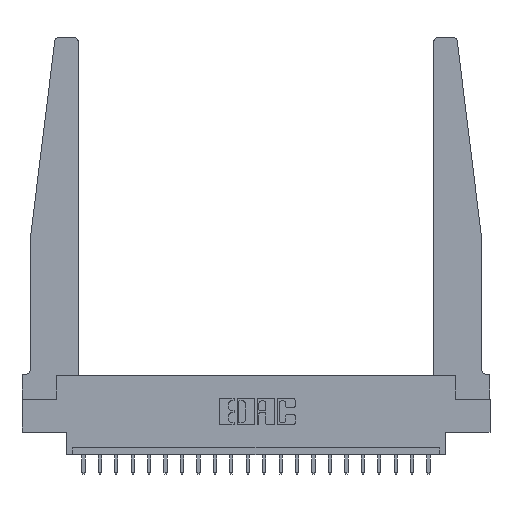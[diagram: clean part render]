
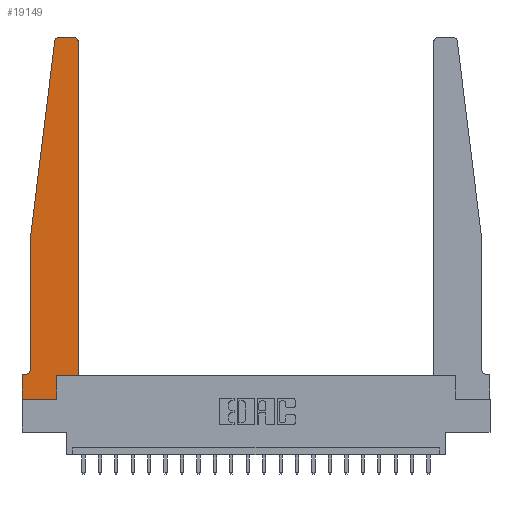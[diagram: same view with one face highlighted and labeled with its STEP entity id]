
A CAD part, top view. The second image highlights one B-rep face of the part: STEP entity #19149.
In plain terms, the highlighted planar face has unit normal (0, 0, 1).
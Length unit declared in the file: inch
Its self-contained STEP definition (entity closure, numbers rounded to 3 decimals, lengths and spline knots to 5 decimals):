
#135 = DIRECTION ( 'NONE',  ( 0., -1., 0. ) ) ;
#217 = ORIENTED_EDGE ( 'NONE', *, *, #11594, .T. ) ;
#1072 = EDGE_CURVE ( 'NONE', #12486, #4913, #5628, .T. ) ;
#1223 = ORIENTED_EDGE ( 'NONE', *, *, #2847, .T. ) ;
#1308 = CARTESIAN_POINT ( 'NONE',  ( 0.065, 0.2375, 0.37 ) ) ;
#1382 = LINE ( 'NONE', #15746, #2912 ) ;
#1485 = LINE ( 'NONE', #18086, #12271 ) ;
#2259 = EDGE_CURVE ( 'NONE', #8871, #21013, #1382, .T. ) ;
#2644 = VECTOR ( 'NONE', #6236, 39.37008 ) ;
#2665 = DIRECTION ( 'NONE',  ( 1., 0., 0. ) ) ;
#2669 = AXIS2_PLACEMENT_3D ( 'NONE', #3501, #15025, #10392 ) ;
#2847 = EDGE_CURVE ( 'NONE', #19261, #7561, #9054, .T. ) ;
#2912 = VECTOR ( 'NONE', #2665, 39.37008 ) ;
#3026 = EDGE_CURVE ( 'NONE', #7064, #3245, #9560, .T. ) ;
#3198 = CARTESIAN_POINT ( 'NONE',  ( 0.24675, 2.72367, 0.37 ) ) ;
#3245 = VERTEX_POINT ( 'NONE', #12214 ) ;
#3501 = CARTESIAN_POINT ( 'NONE',  ( 0.27653, 2.72, 0.37 ) ) ;
#4122 = LINE ( 'NONE', #7102, #8521 ) ;
#4364 = CARTESIAN_POINT ( 'NONE',  ( 0.425, 0.18, 0.37 ) ) ;
#4913 = VERTEX_POINT ( 'NONE', #14708 ) ;
#4915 = DIRECTION ( 'NONE',  ( 0., 0., -1. ) ) ;
#5219 = VERTEX_POINT ( 'NONE', #1308 ) ;
#5628 = LINE ( 'NONE', #20879, #20015 ) ;
#6236 = DIRECTION ( 'NONE',  ( 0., 1., 0. ) ) ;
#6608 = ORIENTED_EDGE ( 'NONE', *, *, #3026, .T. ) ;
#6742 = VECTOR ( 'NONE', #10210, 39.37008 ) ;
#6780 = ORIENTED_EDGE ( 'NONE', *, *, #20189, .T. ) ;
#7064 = VERTEX_POINT ( 'NONE', #3198 ) ;
#7102 = CARTESIAN_POINT ( 'NONE',  ( 0.065, 0.1875, 0.37 ) ) ;
#7144 = CARTESIAN_POINT ( 'NONE',  ( 0.425, 2.72, 0.37 ) ) ;
#7561 = VERTEX_POINT ( 'NONE', #20354 ) ;
#7652 = AXIS2_PLACEMENT_3D ( 'NONE', #14944, #11696, #16441 ) ;
#7834 = ORIENTED_EDGE ( 'NONE', *, *, #17759, .T. ) ;
#8238 = DIRECTION ( 'NONE',  ( 1., 0., 0. ) ) ;
#8492 = CARTESIAN_POINT ( 'NONE',  ( 0.015, 0.1875, 0.37 ) ) ;
#8521 = VECTOR ( 'NONE', #11945, 39.37008 ) ;
#8651 = EDGE_CURVE ( 'NONE', #21013, #19261, #9976, .T. ) ;
#8871 = VERTEX_POINT ( 'NONE', #14206 ) ;
#8902 = EDGE_CURVE ( 'NONE', #5219, #15879, #19164, .T. ) ;
#9054 = CIRCLE ( 'NONE', #15491, 0.03 ) ;
#9259 = DIRECTION ( 'NONE',  ( -1., 0., 0. ) ) ;
#9560 = LINE ( 'NONE', #20122, #6742 ) ;
#9637 = ORIENTED_EDGE ( 'NONE', *, *, #8902, .T. ) ;
#9726 = VECTOR ( 'NONE', #12309, 39.37008 ) ;
#9873 = DIRECTION ( 'NONE',  ( 0., 0., 1. ) ) ;
#9933 = DIRECTION ( 'NONE',  ( -1., 0., 0. ) ) ;
#9976 = LINE ( 'NONE', #10567, #9726 ) ;
#10210 = DIRECTION ( 'NONE',  ( -0.122, -0.992, 0. ) ) ;
#10392 = DIRECTION ( 'NONE',  ( 1., 0., 0. ) ) ;
#10567 = CARTESIAN_POINT ( 'NONE',  ( 0.425, 0.18, 0.37 ) ) ;
#11040 = LINE ( 'NONE', #17439, #18971 ) ;
#11268 = EDGE_CURVE ( 'NONE', #4913, #8871, #11399, .T. ) ;
#11399 = LINE ( 'NONE', #12800, #2644 ) ;
#11484 = PLANE ( 'NONE',  #7652 ) ;
#11594 = EDGE_CURVE ( 'NONE', #18854, #12486, #19063, .T. ) ;
#11696 = DIRECTION ( 'NONE',  ( 0., 0., 1. ) ) ;
#11792 = DIRECTION ( 'NONE',  ( 0., -1., 0. ) ) ;
#11945 = DIRECTION ( 'NONE',  ( -1., 0., 0. ) ) ;
#12076 = FACE_OUTER_BOUND ( 'NONE', #20095, .T. ) ;
#12214 = CARTESIAN_POINT ( 'NONE',  ( 0.065, 1.25, 0.37 ) ) ;
#12271 = VECTOR ( 'NONE', #11792, 39.37008 ) ;
#12309 = DIRECTION ( 'NONE',  ( 0., 1., 0. ) ) ;
#12486 = VERTEX_POINT ( 'NONE', #14514 ) ;
#12800 = CARTESIAN_POINT ( 'NONE',  ( 0.2605, 0.18, 0.37 ) ) ;
#13086 = VERTEX_POINT ( 'NONE', #14207 ) ;
#13185 = VECTOR ( 'NONE', #135, 39.37008 ) ;
#13651 = AXIS2_PLACEMENT_3D ( 'NONE', #15060, #4915, #9933 ) ;
#13880 = EDGE_CURVE ( 'NONE', #13086, #7064, #18957, .T. ) ;
#14080 = ORIENTED_EDGE ( 'NONE', *, *, #8651, .T. ) ;
#14206 = CARTESIAN_POINT ( 'NONE',  ( 0.2605, 0.18, 0.37 ) ) ;
#14207 = CARTESIAN_POINT ( 'NONE',  ( 0.27653, 2.75, 0.37 ) ) ;
#14514 = CARTESIAN_POINT ( 'NONE',  ( 0., 0., 0.37 ) ) ;
#14708 = CARTESIAN_POINT ( 'NONE',  ( 0.2605, 0., 0.37 ) ) ;
#14864 = ORIENTED_EDGE ( 'NONE', *, *, #1072, .T. ) ;
#14944 = CARTESIAN_POINT ( 'NONE',  ( 0., 0.1875, 0.37 ) ) ;
#15025 = DIRECTION ( 'NONE',  ( 0., 0., 1. ) ) ;
#15060 = CARTESIAN_POINT ( 'NONE',  ( 0.015, 0.2375, 0.37 ) ) ;
#15491 = AXIS2_PLACEMENT_3D ( 'NONE', #17991, #9873, #8238 ) ;
#15746 = CARTESIAN_POINT ( 'NONE',  ( 0.425, 0.18, 0.37 ) ) ;
#15879 = VERTEX_POINT ( 'NONE', #8492 ) ;
#16026 = ORIENTED_EDGE ( 'NONE', *, *, #18892, .T. ) ;
#16127 = DIRECTION ( 'NONE',  ( 1., 0., 0. ) ) ;
#16441 = DIRECTION ( 'NONE',  ( 1., 0., 0. ) ) ;
#16693 = CARTESIAN_POINT ( 'NONE',  ( 0., 0., 0.37 ) ) ;
#16878 = ORIENTED_EDGE ( 'NONE', *, *, #11268, .T. ) ;
#17439 = CARTESIAN_POINT ( 'NONE',  ( 0.25, 2.75, 0.37 ) ) ;
#17759 = EDGE_CURVE ( 'NONE', #15879, #18854, #4122, .T. ) ;
#17866 = ORIENTED_EDGE ( 'NONE', *, *, #13880, .T. ) ;
#17991 = CARTESIAN_POINT ( 'NONE',  ( 0.395, 2.72, 0.37 ) ) ;
#18086 = CARTESIAN_POINT ( 'NONE',  ( 0.065, 1.25, 0.37 ) ) ;
#18854 = VERTEX_POINT ( 'NONE', #19252 ) ;
#18892 = EDGE_CURVE ( 'NONE', #7561, #13086, #11040, .T. ) ;
#18957 = CIRCLE ( 'NONE', #2669, 0.03 ) ;
#18971 = VECTOR ( 'NONE', #9259, 39.37008 ) ;
#19063 = LINE ( 'NONE', #16693, #13185 ) ;
#19149 = ADVANCED_FACE ( 'NONE', ( #12076 ), #11484, .T. ) ;
#19164 = CIRCLE ( 'NONE', #13651, 0.05 ) ;
#19252 = CARTESIAN_POINT ( 'NONE',  ( 0., 0.1875, 0.37 ) ) ;
#19261 = VERTEX_POINT ( 'NONE', #7144 ) ;
#20015 = VECTOR ( 'NONE', #16127, 39.37008 ) ;
#20095 = EDGE_LOOP ( 'NONE', ( #16026, #17866, #6608, #6780, #9637, #7834, #217, #14864, #16878, #20309, #14080, #1223 ) ) ;
#20122 = CARTESIAN_POINT ( 'NONE',  ( 0.065, 1.25, 0.37 ) ) ;
#20189 = EDGE_CURVE ( 'NONE', #3245, #5219, #1485, .T. ) ;
#20309 = ORIENTED_EDGE ( 'NONE', *, *, #2259, .T. ) ;
#20354 = CARTESIAN_POINT ( 'NONE',  ( 0.395, 2.75, 0.37 ) ) ;
#20879 = CARTESIAN_POINT ( 'NONE',  ( 0., 0., 0.37 ) ) ;
#21013 = VERTEX_POINT ( 'NONE', #4364 ) ;
